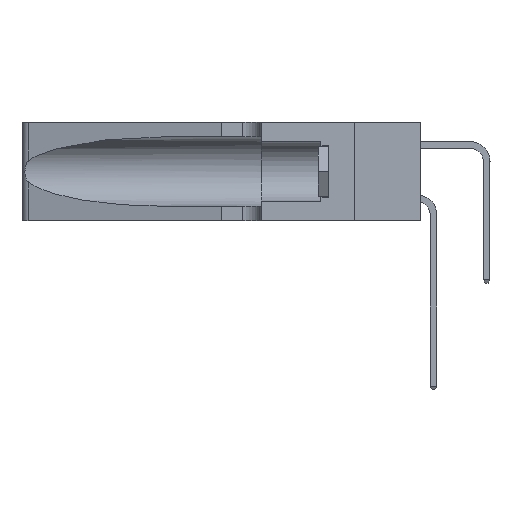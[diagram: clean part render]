
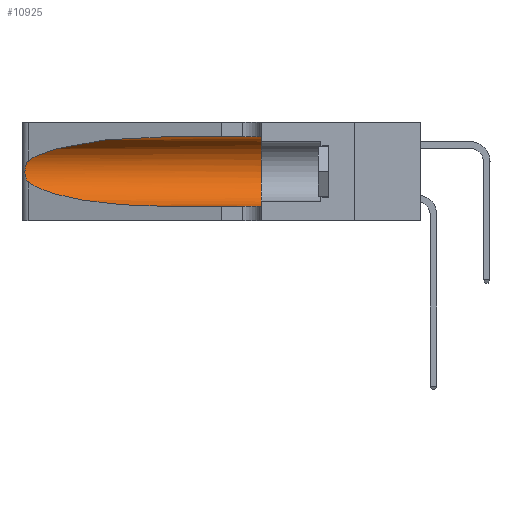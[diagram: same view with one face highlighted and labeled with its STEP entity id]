
A CAD part, left-side view. The second image highlights one B-rep face of the part: STEP entity #10925.
In plain terms, the highlighted cylindrical face has radius 3.308 mm (diameter 6.617 mm), a partial arc.
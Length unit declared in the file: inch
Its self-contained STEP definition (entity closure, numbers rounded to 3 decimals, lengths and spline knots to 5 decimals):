
#45 =( BOUNDED_CURVE ( )  B_SPLINE_CURVE ( 3, ( #17468, #22744, #13816, #17244 ),
 .UNSPECIFIED., .F., .T. ) 
 B_SPLINE_CURVE_WITH_KNOTS ( ( 4, 4 ),
 ( 1.5708, 2.84003 ),
 .UNSPECIFIED. ) 
 CURVE ( )  GEOMETRIC_REPRESENTATION_ITEM ( )  RATIONAL_B_SPLINE_CURVE ( ( 1., 0.87, 0.87, 1. ) ) 
 REPRESENTATION_ITEM ( '' )  );
#119 = CARTESIAN_POINT ( 'NONE',  ( 0.1305, 0.72297, 0.05475 ) ) ;
#203 = CARTESIAN_POINT ( 'NONE',  ( 0.25789, 1.23486, 0.15765 ) ) ;
#211 = VECTOR ( 'NONE', #4068, 39.37008 ) ;
#332 =( BOUNDED_CURVE ( )  B_SPLINE_CURVE ( 3, ( #1843, #19780, #8835, #1688 ),
 .UNSPECIFIED., .F., .F. ) 
 B_SPLINE_CURVE_WITH_KNOTS ( ( 4, 4 ),
 ( 3.44316, 4.71239 ),
 .UNSPECIFIED. ) 
 CURVE ( )  GEOMETRIC_REPRESENTATION_ITEM ( )  RATIONAL_B_SPLINE_CURVE ( ( 1., 0.87, 0.87, 1. ) ) 
 REPRESENTATION_ITEM ( '' )  );
#345 = VERTEX_POINT ( 'NONE', #13447 ) ;
#944 = VERTEX_POINT ( 'NONE', #4417 ) ;
#1680 = EDGE_CURVE ( 'NONE', #345, #5124, #20000, .T. ) ;
#1688 = CARTESIAN_POINT ( 'NONE',  ( 0.1305, 0.72297, 0.05475 ) ) ;
#1843 = CARTESIAN_POINT ( 'NONE',  ( 0.25487, 1.22718, 0.14631 ) ) ;
#1905 = CARTESIAN_POINT ( 'NONE',  ( 0.25854, 1.2359, 0.20912 ) ) ;
#2261 = CARTESIAN_POINT ( 'NONE',  ( 0.1305, 1.61858, 0.05475 ) ) ;
#2405 = CARTESIAN_POINT ( 'NONE',  ( 0.1305, 1.61858, 0.31525 ) ) ;
#2838 = CARTESIAN_POINT ( 'NONE',  ( 0.1305, 0.35, 0.05475 ) ) ;
#4068 = DIRECTION ( 'NONE',  ( 0., -1., 0. ) ) ;
#4129 = EDGE_CURVE ( 'NONE', #9487, #9461, #15252, .T. ) ;
#4328 = DIRECTION ( 'NONE',  ( 0., -1., 0. ) ) ;
#4417 = CARTESIAN_POINT ( 'NONE',  ( 0.1305, 0.72297, 0.31525 ) ) ;
#4851 = ORIENTED_EDGE ( 'NONE', *, *, #1680, .F. ) ;
#5124 = VERTEX_POINT ( 'NONE', #2838 ) ;
#5245 = LINE ( 'NONE', #2405, #211 ) ;
#5354 = ORIENTED_EDGE ( 'NONE', *, *, #20784, .T. ) ;
#5530 = CARTESIAN_POINT ( 'NONE',  ( 0.26018, 1.23835, 0.19895 ) ) ;
#5833 = CARTESIAN_POINT ( 'NONE',  ( 0.1305, 1.61858, 0.185 ) ) ;
#6430 = LINE ( 'NONE', #2261, #13462 ) ;
#7027 = CARTESIAN_POINT ( 'NONE',  ( 0.26075, 1.23896, 0.178 ) ) ;
#7191 = CARTESIAN_POINT ( 'NONE',  ( 0.26075, 1.23896, 0.19203 ) ) ;
#7345 = CARTESIAN_POINT ( 'NONE',  ( 0.26017, 1.23833, 0.17102 ) ) ;
#7757 = ORIENTED_EDGE ( 'NONE', *, *, #12977, .F. ) ;
#8278 = ORIENTED_EDGE ( 'NONE', *, *, #10179, .T. ) ;
#8717 = CARTESIAN_POINT ( 'NONE',  ( 0.25487, 1.22718, 0.14631 ) ) ;
#8835 = CARTESIAN_POINT ( 'NONE',  ( 0.18966, 0.96281, 0.05475 ) ) ;
#9143 = CARTESIAN_POINT ( 'NONE',  ( 0.25856, 1.23593, 0.16098 ) ) ;
#9461 = VERTEX_POINT ( 'NONE', #8717 ) ;
#9487 = VERTEX_POINT ( 'NONE', #19493 ) ;
#10179 = EDGE_CURVE ( 'NONE', #9461, #13549, #332, .T. ) ;
#10723 = CARTESIAN_POINT ( 'NONE',  ( 0.25639, 1.23186, 0.15144 ) ) ;
#10882 = CARTESIAN_POINT ( 'NONE',  ( 0.25555, 1.22994, 0.2215 ) ) ;
#10925 = ADVANCED_FACE ( 'NONE', ( #12125 ), #13528, .F. ) ;
#11283 = AXIS2_PLACEMENT_3D ( 'NONE', #5833, #14829, #13135 ) ;
#12125 = FACE_OUTER_BOUND ( 'NONE', #16100, .T. ) ;
#12977 = EDGE_CURVE ( 'NONE', #944, #345, #5245, .T. ) ;
#13135 = DIRECTION ( 'NONE',  ( 0., 0., -1. ) ) ;
#13447 = CARTESIAN_POINT ( 'NONE',  ( 0.1305, 0.35, 0.31525 ) ) ;
#13462 = VECTOR ( 'NONE', #4328, 39.37008 ) ;
#13528 = CYLINDRICAL_SURFACE ( 'NONE', #11283, 0.13025 ) ;
#13549 = VERTEX_POINT ( 'NONE', #119 ) ;
#13780 = CARTESIAN_POINT ( 'NONE',  ( 0.1305, 0.35, 0.185 ) ) ;
#13816 = CARTESIAN_POINT ( 'NONE',  ( 0.2373, 1.15595, 0.28018 ) ) ;
#14829 = DIRECTION ( 'NONE',  ( 0., -1., 0. ) ) ;
#15252 = B_SPLINE_CURVE_WITH_KNOTS ( 'NONE', 3,
 ( #21391, #10882, #17810, #18046, #1905, #5530, #7191, #7027, #7345, #9143, #203, #10723, #21625, #21312 ),
 .UNSPECIFIED., .F., .F.,
 ( 4, 2, 2, 2, 2, 2, 4 ),
 ( 0., 0.00027, 0.00053, 0.00107, 0.0016, 0.00187, 0.00214 ),
 .UNSPECIFIED. ) ;
#16100 = EDGE_LOOP ( 'NONE', ( #18072, #21083, #8278, #5354, #4851, #7757 ) ) ;
#17244 = CARTESIAN_POINT ( 'NONE',  ( 0.25487, 1.22718, 0.22369 ) ) ;
#17468 = CARTESIAN_POINT ( 'NONE',  ( 0.1305, 0.72297, 0.31525 ) ) ;
#17661 = DIRECTION ( 'NONE',  ( 0., 1., 0. ) ) ;
#17780 = EDGE_CURVE ( 'NONE', #944, #9487, #45, .T. ) ;
#17810 = CARTESIAN_POINT ( 'NONE',  ( 0.25639, 1.23184, 0.21858 ) ) ;
#18046 = CARTESIAN_POINT ( 'NONE',  ( 0.25787, 1.23484, 0.2124 ) ) ;
#18072 = ORIENTED_EDGE ( 'NONE', *, *, #17780, .T. ) ;
#18740 = AXIS2_PLACEMENT_3D ( 'NONE', #13780, #17661, #19704 ) ;
#19493 = CARTESIAN_POINT ( 'NONE',  ( 0.25487, 1.22718, 0.22369 ) ) ;
#19704 = DIRECTION ( 'NONE',  ( 0., 0., 1. ) ) ;
#19780 = CARTESIAN_POINT ( 'NONE',  ( 0.2373, 1.15595, 0.08982 ) ) ;
#20000 = CIRCLE ( 'NONE', #18740, 0.13025 ) ;
#20784 = EDGE_CURVE ( 'NONE', #13549, #5124, #6430, .T. ) ;
#21083 = ORIENTED_EDGE ( 'NONE', *, *, #4129, .T. ) ;
#21312 = CARTESIAN_POINT ( 'NONE',  ( 0.25487, 1.22718, 0.14631 ) ) ;
#21391 = CARTESIAN_POINT ( 'NONE',  ( 0.25487, 1.22718, 0.22369 ) ) ;
#21625 = CARTESIAN_POINT ( 'NONE',  ( 0.25555, 1.22993, 0.14849 ) ) ;
#22744 = CARTESIAN_POINT ( 'NONE',  ( 0.18966, 0.96281, 0.31525 ) ) ;
